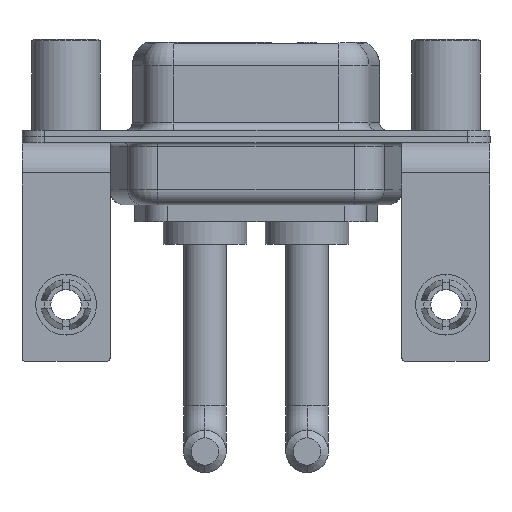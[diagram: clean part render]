
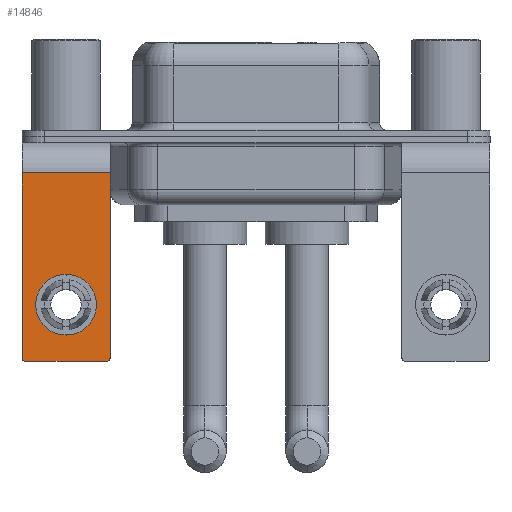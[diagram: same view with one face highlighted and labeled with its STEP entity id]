
A CAD part, front view. The second image highlights one B-rep face of the part: STEP entity #14846.
In plain terms, the highlighted planar face has unit normal (0, -1, 0).
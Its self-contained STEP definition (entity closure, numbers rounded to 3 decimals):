
#54 = ORIENTED_EDGE ( 'NONE', *, *, #6099, .T. ) ;
#287 = CARTESIAN_POINT ( 'NONE',  ( 2.9, -6.25, -2.4 ) ) ;
#565 = CARTESIAN_POINT ( 'NONE',  ( 2.65, -6.25, -14.8 ) ) ;
#1011 = PLANE ( 'NONE',  #3233 ) ;
#1643 = CARTESIAN_POINT ( 'NONE',  ( -2.9, -6.25, -14.55 ) ) ;
#1666 = VECTOR ( 'NONE', #8994, 1000. ) ;
#2080 = CARTESIAN_POINT ( 'NONE',  ( 2.9, -6.25, -2.4 ) ) ;
#2329 = EDGE_CURVE ( 'NONE', #3172, #9537, #4255, .T. ) ;
#2950 = LINE ( 'NONE', #287, #8736 ) ;
#2975 = ORIENTED_EDGE ( 'NONE', *, *, #6079, .T. ) ;
#3009 = DIRECTION ( 'NONE',  ( 0., 0., 1. ) ) ;
#3172 = VERTEX_POINT ( 'NONE', #8628 ) ;
#3233 = AXIS2_PLACEMENT_3D ( 'NONE', #2080, #13108, #6391 ) ;
#3587 = VERTEX_POINT ( 'NONE', #9489 ) ;
#4255 = CIRCLE ( 'NONE', #14684, 2. ) ;
#4277 = CIRCLE ( 'NONE', #6530, 0.25 ) ;
#4304 = LINE ( 'NONE', #8379, #9120 ) ;
#4668 = DIRECTION ( 'NONE',  ( 0., 1., 0. ) ) ;
#5192 = VECTOR ( 'NONE', #12222, 1000. ) ;
#5281 = VERTEX_POINT ( 'NONE', #5505 ) ;
#5505 = CARTESIAN_POINT ( 'NONE',  ( 2.9, -6.25, -2.4 ) ) ;
#5650 = AXIS2_PLACEMENT_3D ( 'NONE', #15739, #10609, #7706 ) ;
#6079 = EDGE_CURVE ( 'NONE', #9537, #3172, #12387, .T. ) ;
#6099 = EDGE_CURVE ( 'NONE', #5281, #3587, #17029, .T. ) ;
#6391 = DIRECTION ( 'NONE',  ( 0., 0., 1. ) ) ;
#6530 = AXIS2_PLACEMENT_3D ( 'NONE', #10750, #13657, #12421 ) ;
#6703 = EDGE_LOOP ( 'NONE', ( #13262, #2975 ) ) ;
#6833 = CARTESIAN_POINT ( 'NONE',  ( -2.9, -6.25, -2.4 ) ) ;
#6893 = ORIENTED_EDGE ( 'NONE', *, *, #14116, .T. ) ;
#6913 = VERTEX_POINT ( 'NONE', #17053 ) ;
#7028 = AXIS2_PLACEMENT_3D ( 'NONE', #13058, #4668, #9082 ) ;
#7190 = ORIENTED_EDGE ( 'NONE', *, *, #8912, .T. ) ;
#7215 = VERTEX_POINT ( 'NONE', #565 ) ;
#7706 = DIRECTION ( 'NONE',  ( 0., 0., 1. ) ) ;
#8379 = CARTESIAN_POINT ( 'NONE',  ( 2.9, -6.25, -14.8 ) ) ;
#8432 = DIRECTION ( 'NONE',  ( 0., 0., -1. ) ) ;
#8628 = CARTESIAN_POINT ( 'NONE',  ( 0., -6.25, -13.07 ) ) ;
#8736 = VECTOR ( 'NONE', #8432, 1000. ) ;
#8912 = EDGE_CURVE ( 'NONE', #16019, #6913, #11571, .T. ) ;
#8994 = DIRECTION ( 'NONE',  ( -1., 0., 0. ) ) ;
#9082 = DIRECTION ( 'NONE',  ( 0., 0., 1. ) ) ;
#9120 = VECTOR ( 'NONE', #13743, 1000. ) ;
#9489 = CARTESIAN_POINT ( 'NONE',  ( -2.9, -6.25, -2.4 ) ) ;
#9537 = VERTEX_POINT ( 'NONE', #10856 ) ;
#9726 = CARTESIAN_POINT ( 'NONE',  ( 0., -6.25, -11.07 ) ) ;
#9826 = LINE ( 'NONE', #6833, #5192 ) ;
#10252 = EDGE_CURVE ( 'NONE', #7215, #11859, #4277, .T. ) ;
#10609 = DIRECTION ( 'NONE',  ( 0., -1., 0. ) ) ;
#10750 = CARTESIAN_POINT ( 'NONE',  ( 2.65, -6.25, -14.55 ) ) ;
#10856 = CARTESIAN_POINT ( 'NONE',  ( 0., -6.25, -9.07 ) ) ;
#11519 = FACE_BOUND ( 'NONE', #6703, .T. ) ;
#11550 = CARTESIAN_POINT ( 'NONE',  ( 2.9, -6.25, -2.4 ) ) ;
#11571 = CIRCLE ( 'NONE', #5650, 0.25 ) ;
#11859 = VERTEX_POINT ( 'NONE', #16745 ) ;
#12222 = DIRECTION ( 'NONE',  ( 0., 0., -1. ) ) ;
#12387 = CIRCLE ( 'NONE', #7028, 2. ) ;
#12421 = DIRECTION ( 'NONE',  ( 0., 0., 1. ) ) ;
#13058 = CARTESIAN_POINT ( 'NONE',  ( 0., -6.25, -11.07 ) ) ;
#13108 = DIRECTION ( 'NONE',  ( 0., 1., 0. ) ) ;
#13135 = EDGE_CURVE ( 'NONE', #7215, #6913, #4304, .T. ) ;
#13262 = ORIENTED_EDGE ( 'NONE', *, *, #2329, .T. ) ;
#13657 = DIRECTION ( 'NONE',  ( 0., -1., 0. ) ) ;
#13743 = DIRECTION ( 'NONE',  ( -1., 0., 0. ) ) ;
#14116 = EDGE_CURVE ( 'NONE', #3587, #16019, #9826, .T. ) ;
#14400 = ORIENTED_EDGE ( 'NONE', *, *, #13135, .F. ) ;
#14684 = AXIS2_PLACEMENT_3D ( 'NONE', #9726, #15115, #3009 ) ;
#14846 = ADVANCED_FACE ( 'NONE', ( #11519, #15761 ), #1011, .F. ) ;
#14851 = EDGE_LOOP ( 'NONE', ( #6893, #7190, #14400, #16809, #15895, #54 ) ) ;
#15115 = DIRECTION ( 'NONE',  ( 0., 1., 0. ) ) ;
#15297 = EDGE_CURVE ( 'NONE', #5281, #11859, #2950, .T. ) ;
#15739 = CARTESIAN_POINT ( 'NONE',  ( -2.65, -6.25, -14.55 ) ) ;
#15761 = FACE_OUTER_BOUND ( 'NONE', #14851, .T. ) ;
#15895 = ORIENTED_EDGE ( 'NONE', *, *, #15297, .F. ) ;
#16019 = VERTEX_POINT ( 'NONE', #1643 ) ;
#16745 = CARTESIAN_POINT ( 'NONE',  ( 2.9, -6.25, -14.55 ) ) ;
#16809 = ORIENTED_EDGE ( 'NONE', *, *, #10252, .T. ) ;
#17029 = LINE ( 'NONE', #11550, #1666 ) ;
#17053 = CARTESIAN_POINT ( 'NONE',  ( -2.65, -6.25, -14.8 ) ) ;
